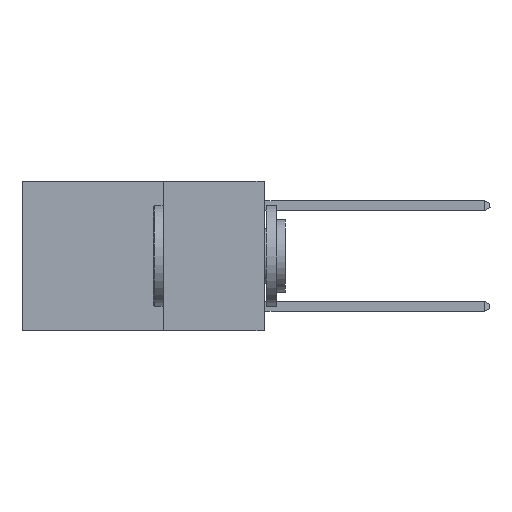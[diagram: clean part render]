
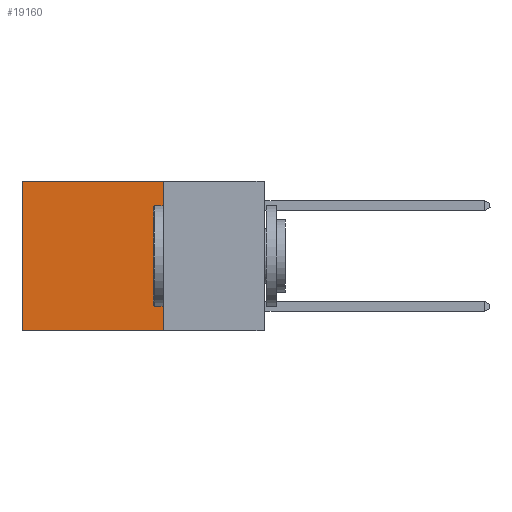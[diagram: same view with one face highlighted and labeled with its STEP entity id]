
A CAD part, left-side view. The second image highlights one B-rep face of the part: STEP entity #19160.
In plain terms, the highlighted planar face has unit normal (-1, 0, 0).
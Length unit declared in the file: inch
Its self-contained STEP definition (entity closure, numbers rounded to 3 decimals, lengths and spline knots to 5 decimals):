
#12 = PLANE ( 'NONE',  #19036 ) ;
#1399 = LINE ( 'NONE', #18450, #6956 ) ;
#1992 = CARTESIAN_POINT ( 'NONE',  ( 0.2625, 0.6, -0.37 ) ) ;
#2106 = EDGE_CURVE ( 'NONE', #13555, #27363, #1399, .T. ) ;
#4133 = EDGE_CURVE ( 'NONE', #20443, #13555, #29011, .T. ) ;
#4240 = FACE_OUTER_BOUND ( 'NONE', #5610, .T. ) ;
#4477 = DIRECTION ( 'NONE',  ( 0., 0., -1. ) ) ;
#4820 = DIRECTION ( 'NONE',  ( 0., 0., -1. ) ) ;
#5308 = VECTOR ( 'NONE', #8846, 39.37008 ) ;
#5610 = EDGE_LOOP ( 'NONE', ( #8188, #16883, #13366, #8559 ) ) ;
#5763 = VERTEX_POINT ( 'NONE', #10342 ) ;
#6673 = EDGE_CURVE ( 'NONE', #20443, #5763, #27807, .T. ) ;
#6956 = VECTOR ( 'NONE', #4477, 39.37008 ) ;
#8188 = ORIENTED_EDGE ( 'NONE', *, *, #2106, .T. ) ;
#8559 = ORIENTED_EDGE ( 'NONE', *, *, #4133, .T. ) ;
#8846 = DIRECTION ( 'NONE',  ( 0., 1., 0. ) ) ;
#9582 = CARTESIAN_POINT ( 'NONE',  ( 0.2625, 0.25, 0. ) ) ;
#9827 = CARTESIAN_POINT ( 'NONE',  ( 0.2625, 0.25, 0. ) ) ;
#10342 = CARTESIAN_POINT ( 'NONE',  ( 0.2625, 0.25, -0.37 ) ) ;
#11513 = CARTESIAN_POINT ( 'NONE',  ( 0.2625, 0.25, 0. ) ) ;
#13002 = LINE ( 'NONE', #18186, #5308 ) ;
#13366 = ORIENTED_EDGE ( 'NONE', *, *, #6673, .F. ) ;
#13555 = VERTEX_POINT ( 'NONE', #17996 ) ;
#13647 = EDGE_CURVE ( 'NONE', #5763, #27363, #13002, .T. ) ;
#16471 = CARTESIAN_POINT ( 'NONE',  ( 0.2625, 0.25, 0. ) ) ;
#16883 = ORIENTED_EDGE ( 'NONE', *, *, #13647, .F. ) ;
#17996 = CARTESIAN_POINT ( 'NONE',  ( 0.2625, 0.6, 0. ) ) ;
#18186 = CARTESIAN_POINT ( 'NONE',  ( 0.2625, 0.25, -0.37 ) ) ;
#18450 = CARTESIAN_POINT ( 'NONE',  ( 0.2625, 0.6, 0. ) ) ;
#18511 = DIRECTION ( 'NONE',  ( 0., 0., -1. ) ) ;
#18787 = DIRECTION ( 'NONE',  ( 1., 0., 0. ) ) ;
#19036 = AXIS2_PLACEMENT_3D ( 'NONE', #16471, #18787, #4820 ) ;
#19160 = ADVANCED_FACE ( 'NONE', ( #4240 ), #12, .F. ) ;
#20443 = VERTEX_POINT ( 'NONE', #9582 ) ;
#21442 = VECTOR ( 'NONE', #23799, 39.37008 ) ;
#21669 = VECTOR ( 'NONE', #18511, 39.37008 ) ;
#23799 = DIRECTION ( 'NONE',  ( 0., 1., 0. ) ) ;
#27363 = VERTEX_POINT ( 'NONE', #1992 ) ;
#27807 = LINE ( 'NONE', #11513, #21669 ) ;
#29011 = LINE ( 'NONE', #9827, #21442 ) ;
